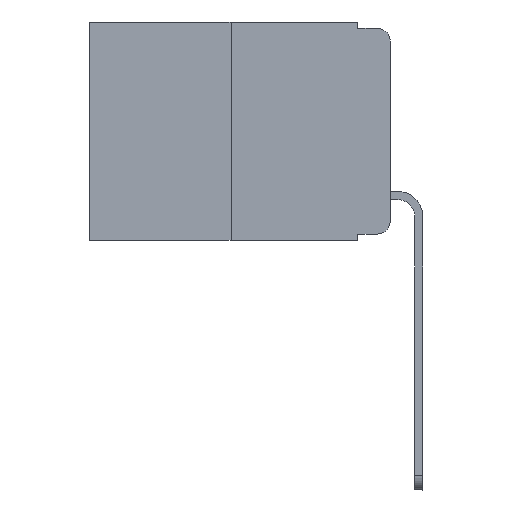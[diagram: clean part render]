
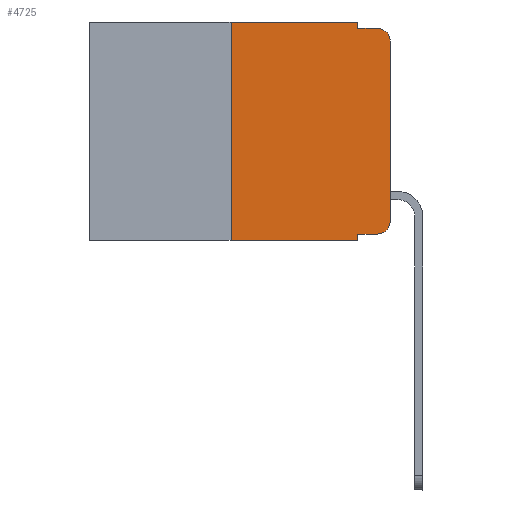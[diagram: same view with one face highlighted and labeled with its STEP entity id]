
A CAD part, left-side view. The second image highlights one B-rep face of the part: STEP entity #4725.
In plain terms, the highlighted planar face has unit normal (-1, 0, 0).
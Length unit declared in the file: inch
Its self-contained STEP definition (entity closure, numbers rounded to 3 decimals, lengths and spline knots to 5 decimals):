
#823 = CARTESIAN_POINT ( 'NONE',  ( 0., 0.02, -0.01 ) ) ;
#1132 = EDGE_CURVE ( 'NONE', #23048, #11495, #2173, .T. ) ;
#1216 = CARTESIAN_POINT ( 'NONE',  ( 0., 0.473, 0. ) ) ;
#1446 = CARTESIAN_POINT ( 'NONE',  ( 0., 0.473, 0. ) ) ;
#1521 = ORIENTED_EDGE ( 'NONE', *, *, #22228, .T. ) ;
#1623 = VERTEX_POINT ( 'NONE', #7556 ) ;
#1801 = ORIENTED_EDGE ( 'NONE', *, *, #1132, .T. ) ;
#2035 = DIRECTION ( 'NONE',  ( 0., 0., -1. ) ) ;
#2173 = CIRCLE ( 'NONE', #9158, 0.02 ) ;
#2489 = CARTESIAN_POINT ( 'NONE',  ( 0., 0.473, -0.343 ) ) ;
#2921 = EDGE_CURVE ( 'NONE', #13246, #12704, #19092, .T. ) ;
#3083 = ORIENTED_EDGE ( 'NONE', *, *, #6042, .F. ) ;
#3187 = CARTESIAN_POINT ( 'NONE',  ( 0., 0.25, -0.343 ) ) ;
#3343 = CARTESIAN_POINT ( 'NONE',  ( 0., 0., -0.03 ) ) ;
#4440 = LINE ( 'NONE', #12079, #15900 ) ;
#4443 = DIRECTION ( 'NONE',  ( 0., -1., 0. ) ) ;
#4453 = AXIS2_PLACEMENT_3D ( 'NONE', #9876, #21187, #15600 ) ;
#4725 = ADVANCED_FACE ( 'NONE', ( #17904 ), #5021, .F. ) ;
#5021 = PLANE ( 'NONE',  #8464 ) ;
#5488 = DIRECTION ( 'NONE',  ( 0., -1., 0. ) ) ;
#5520 = VECTOR ( 'NONE', #4443, 39.37008 ) ;
#5600 = VERTEX_POINT ( 'NONE', #8331 ) ;
#6042 = EDGE_CURVE ( 'NONE', #22661, #5600, #4440, .T. ) ;
#6170 = VERTEX_POINT ( 'NONE', #3343 ) ;
#6501 = CARTESIAN_POINT ( 'NONE',  ( 0., 0., 0. ) ) ;
#6851 = VECTOR ( 'NONE', #12628, 39.37008 ) ;
#6982 = DIRECTION ( 'NONE',  ( -1., 0., 0. ) ) ;
#7556 = CARTESIAN_POINT ( 'NONE',  ( 0., 0.051, -0.333 ) ) ;
#8331 = CARTESIAN_POINT ( 'NONE',  ( 0., 0.25, 0. ) ) ;
#8464 = AXIS2_PLACEMENT_3D ( 'NONE', #1216, #8756, #8873 ) ;
#8639 = ORIENTED_EDGE ( 'NONE', *, *, #9318, .T. ) ;
#8740 = ORIENTED_EDGE ( 'NONE', *, *, #10135, .F. ) ;
#8746 = ORIENTED_EDGE ( 'NONE', *, *, #14419, .F. ) ;
#8756 = DIRECTION ( 'NONE',  ( 1., 0., 0. ) ) ;
#8861 = DIRECTION ( 'NONE',  ( 0., -1., 0. ) ) ;
#8873 = DIRECTION ( 'NONE',  ( 0., 0., -1. ) ) ;
#9158 = AXIS2_PLACEMENT_3D ( 'NONE', #14536, #6982, #16001 ) ;
#9200 = LINE ( 'NONE', #12874, #6851 ) ;
#9318 = EDGE_CURVE ( 'NONE', #6170, #12704, #14945, .T. ) ;
#9876 = CARTESIAN_POINT ( 'NONE',  ( 0., 0.02, -0.03 ) ) ;
#10097 = EDGE_CURVE ( 'NONE', #1623, #23048, #22139, .T. ) ;
#10134 = LINE ( 'NONE', #2489, #5520 ) ;
#10135 = EDGE_CURVE ( 'NONE', #5600, #16621, #11300, .T. ) ;
#11300 = LINE ( 'NONE', #1446, #20626 ) ;
#11495 = VERTEX_POINT ( 'NONE', #13610 ) ;
#11507 = CARTESIAN_POINT ( 'NONE',  ( 0., 0.051, 0. ) ) ;
#11752 = ORIENTED_EDGE ( 'NONE', *, *, #15678, .F. ) ;
#11934 = ORIENTED_EDGE ( 'NONE', *, *, #2921, .F. ) ;
#11951 = VECTOR ( 'NONE', #2035, 39.37008 ) ;
#12079 = CARTESIAN_POINT ( 'NONE',  ( 0., 0.25, 0. ) ) ;
#12101 = DIRECTION ( 'NONE',  ( 0., 0., 1. ) ) ;
#12628 = DIRECTION ( 'NONE',  ( 0., 0., -1. ) ) ;
#12701 = VECTOR ( 'NONE', #17293, 39.37008 ) ;
#12704 = VERTEX_POINT ( 'NONE', #823 ) ;
#12874 = CARTESIAN_POINT ( 'NONE',  ( 0., 0.051, 0. ) ) ;
#13110 = LINE ( 'NONE', #11507, #11951 ) ;
#13246 = VERTEX_POINT ( 'NONE', #19029 ) ;
#13610 = CARTESIAN_POINT ( 'NONE',  ( 0., 0., -0.313 ) ) ;
#13833 = CARTESIAN_POINT ( 'NONE',  ( 0., 0.051, -0.343 ) ) ;
#13843 = CARTESIAN_POINT ( 'NONE',  ( 0., 0.02, -0.333 ) ) ;
#14220 = VERTEX_POINT ( 'NONE', #13833 ) ;
#14419 = EDGE_CURVE ( 'NONE', #1623, #14220, #9200, .T. ) ;
#14536 = CARTESIAN_POINT ( 'NONE',  ( 0., 0.02, -0.313 ) ) ;
#14945 = CIRCLE ( 'NONE', #4453, 0.02 ) ;
#15221 = CARTESIAN_POINT ( 'NONE',  ( 0., 0.051, -0.01 ) ) ;
#15600 = DIRECTION ( 'NONE',  ( 0., 0., -1. ) ) ;
#15632 = LINE ( 'NONE', #6501, #20692 ) ;
#15678 = EDGE_CURVE ( 'NONE', #16621, #13246, #13110, .T. ) ;
#15900 = VECTOR ( 'NONE', #19492, 39.37008 ) ;
#16001 = DIRECTION ( 'NONE',  ( 0., 0., -1. ) ) ;
#16126 = ORIENTED_EDGE ( 'NONE', *, *, #10097, .T. ) ;
#16621 = VERTEX_POINT ( 'NONE', #18524 ) ;
#17293 = DIRECTION ( 'NONE',  ( 0., -1., 0. ) ) ;
#17518 = VECTOR ( 'NONE', #5488, 39.37008 ) ;
#17904 = FACE_OUTER_BOUND ( 'NONE', #22024, .T. ) ;
#18524 = CARTESIAN_POINT ( 'NONE',  ( 0., 0.051, 0. ) ) ;
#19029 = CARTESIAN_POINT ( 'NONE',  ( 0., 0.051, -0.01 ) ) ;
#19092 = LINE ( 'NONE', #15221, #12701 ) ;
#19492 = DIRECTION ( 'NONE',  ( 0., 0., 1. ) ) ;
#19538 = EDGE_CURVE ( 'NONE', #22661, #14220, #10134, .T. ) ;
#20626 = VECTOR ( 'NONE', #8861, 39.37008 ) ;
#20692 = VECTOR ( 'NONE', #12101, 39.37008 ) ;
#21187 = DIRECTION ( 'NONE',  ( -1., 0., 0. ) ) ;
#21880 = ORIENTED_EDGE ( 'NONE', *, *, #19538, .T. ) ;
#22024 = EDGE_LOOP ( 'NONE', ( #1521, #8639, #11934, #11752, #8740, #3083, #21880, #8746, #16126, #1801 ) ) ;
#22139 = LINE ( 'NONE', #23846, #17518 ) ;
#22228 = EDGE_CURVE ( 'NONE', #11495, #6170, #15632, .T. ) ;
#22661 = VERTEX_POINT ( 'NONE', #3187 ) ;
#23048 = VERTEX_POINT ( 'NONE', #13843 ) ;
#23846 = CARTESIAN_POINT ( 'NONE',  ( 0., 0.051, -0.333 ) ) ;
